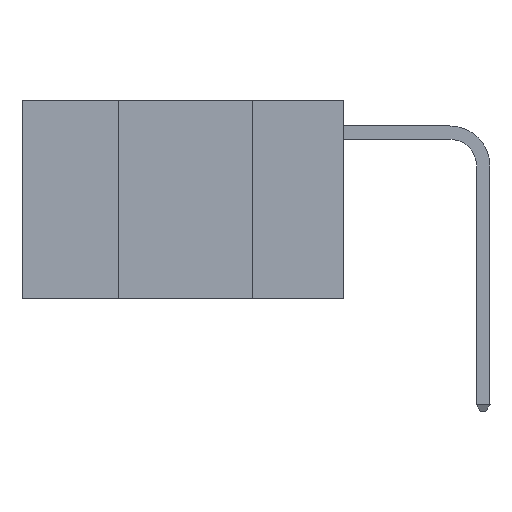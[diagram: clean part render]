
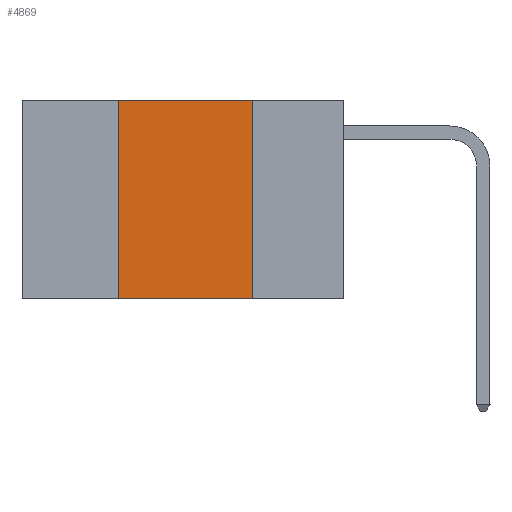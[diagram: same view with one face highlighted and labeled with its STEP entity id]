
A CAD part, left-side view. The second image highlights one B-rep face of the part: STEP entity #4869.
In plain terms, the highlighted planar face has unit normal (-1, 0, 0).
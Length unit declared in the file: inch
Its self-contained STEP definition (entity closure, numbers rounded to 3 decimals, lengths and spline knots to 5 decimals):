
#787 = VECTOR ( 'NONE', #5777, 39.37008 ) ;
#924 = VECTOR ( 'NONE', #8013, 39.37008 ) ;
#1280 = EDGE_CURVE ( 'NONE', #4691, #2036, #2162, .T. ) ;
#1551 = CARTESIAN_POINT ( 'NONE',  ( 0., 0.17, 0. ) ) ;
#1613 = FACE_OUTER_BOUND ( 'NONE', #4812, .T. ) ;
#2016 = VECTOR ( 'NONE', #3735, 39.37008 ) ;
#2036 = VERTEX_POINT ( 'NONE', #9336 ) ;
#2162 = LINE ( 'NONE', #5107, #924 ) ;
#2608 = AXIS2_PLACEMENT_3D ( 'NONE', #6042, #4511, #7423 ) ;
#2793 = CARTESIAN_POINT ( 'NONE',  ( 0., 0.42, -0.37 ) ) ;
#3248 = VECTOR ( 'NONE', #9288, 39.37008 ) ;
#3735 = DIRECTION ( 'NONE',  ( 0., 0., -1. ) ) ;
#3865 = LINE ( 'NONE', #1551, #2016 ) ;
#3987 = VERTEX_POINT ( 'NONE', #6832 ) ;
#4070 = LINE ( 'NONE', #4839, #3248 ) ;
#4511 = DIRECTION ( 'NONE',  ( 1., 0., 0. ) ) ;
#4691 = VERTEX_POINT ( 'NONE', #2793 ) ;
#4812 = EDGE_LOOP ( 'NONE', ( #5689, #6300, #7487, #5234 ) ) ;
#4839 = CARTESIAN_POINT ( 'NONE',  ( 0., 0.6, -0.37 ) ) ;
#4869 = ADVANCED_FACE ( 'NONE', ( #1613 ), #8917, .F. ) ;
#5107 = CARTESIAN_POINT ( 'NONE',  ( 0., 0.42, 0. ) ) ;
#5150 = VERTEX_POINT ( 'NONE', #5713 ) ;
#5234 = ORIENTED_EDGE ( 'NONE', *, *, #6032, .T. ) ;
#5689 = ORIENTED_EDGE ( 'NONE', *, *, #7397, .F. ) ;
#5713 = CARTESIAN_POINT ( 'NONE',  ( 0., 0.17, -0.37 ) ) ;
#5777 = DIRECTION ( 'NONE',  ( 0., -1., 0. ) ) ;
#6032 = EDGE_CURVE ( 'NONE', #4691, #5150, #4070, .T. ) ;
#6042 = CARTESIAN_POINT ( 'NONE',  ( 0., 0.6, 0. ) ) ;
#6300 = ORIENTED_EDGE ( 'NONE', *, *, #7551, .F. ) ;
#6832 = CARTESIAN_POINT ( 'NONE',  ( 0., 0.17, 0. ) ) ;
#7397 = EDGE_CURVE ( 'NONE', #3987, #5150, #3865, .T. ) ;
#7423 = DIRECTION ( 'NONE',  ( 0., 0., -1. ) ) ;
#7487 = ORIENTED_EDGE ( 'NONE', *, *, #1280, .F. ) ;
#7551 = EDGE_CURVE ( 'NONE', #2036, #3987, #8015, .T. ) ;
#8013 = DIRECTION ( 'NONE',  ( 0., 0., 1. ) ) ;
#8015 = LINE ( 'NONE', #8597, #787 ) ;
#8597 = CARTESIAN_POINT ( 'NONE',  ( 0., 0.6, 0. ) ) ;
#8917 = PLANE ( 'NONE',  #2608 ) ;
#9288 = DIRECTION ( 'NONE',  ( 0., -1., 0. ) ) ;
#9336 = CARTESIAN_POINT ( 'NONE',  ( 0., 0.42, 0. ) ) ;
